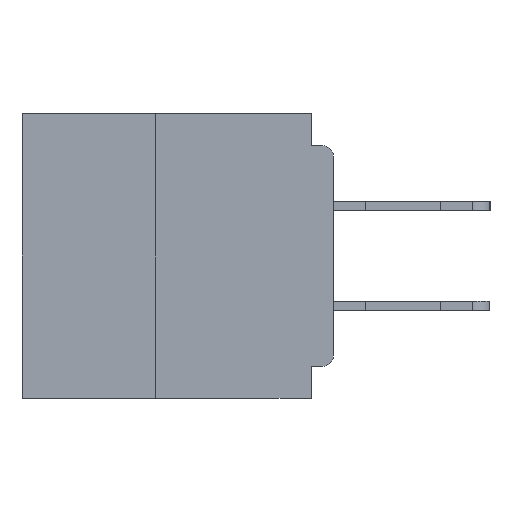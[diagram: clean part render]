
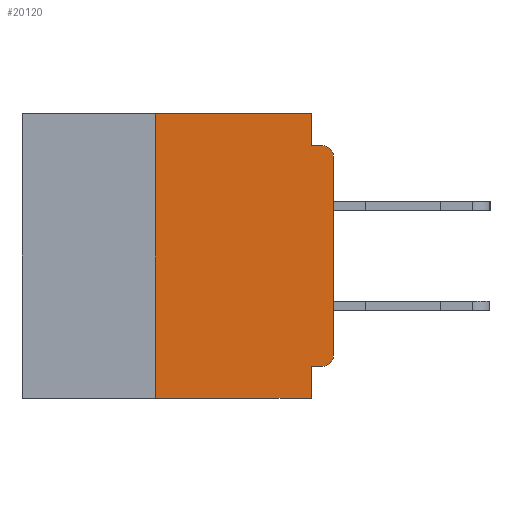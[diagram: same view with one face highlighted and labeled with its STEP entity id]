
A CAD part, left-side view. The second image highlights one B-rep face of the part: STEP entity #20120.
In plain terms, the highlighted planar face has unit normal (-1, 0, 0).
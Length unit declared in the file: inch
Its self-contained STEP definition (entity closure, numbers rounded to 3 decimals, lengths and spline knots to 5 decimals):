
#672 = CARTESIAN_POINT ( 'NONE',  ( 0., 0., -0.06 ) ) ;
#789 = CARTESIAN_POINT ( 'NONE',  ( 0., 0.031, -0.045 ) ) ;
#792 = EDGE_CURVE ( 'NONE', #22441, #14291, #31582, .T. ) ;
#2682 = EDGE_CURVE ( 'NONE', #5539, #14291, #34932, .T. ) ;
#2962 = DIRECTION ( 'NONE',  ( 0., 1., 0. ) ) ;
#2996 = LINE ( 'NONE', #38548, #36678 ) ;
#3114 = EDGE_LOOP ( 'NONE', ( #33244, #31197, #29555, #33017, #8066, #11037, #27765, #27818, #9573, #27859 ) ) ;
#3295 = CARTESIAN_POINT ( 'NONE',  ( 0., 0.437, 0. ) ) ;
#4267 = DIRECTION ( 'NONE',  ( 0., 0., -1. ) ) ;
#4683 = VERTEX_POINT ( 'NONE', #6016 ) ;
#4713 = AXIS2_PLACEMENT_3D ( 'NONE', #6894, #29725, #10182 ) ;
#5215 = VECTOR ( 'NONE', #4267, 39.37008 ) ;
#5427 = DIRECTION ( 'NONE',  ( 0., 0., -1. ) ) ;
#5489 = DIRECTION ( 'NONE',  ( -1., 0., 0. ) ) ;
#5539 = VERTEX_POINT ( 'NONE', #672 ) ;
#5543 = CARTESIAN_POINT ( 'NONE',  ( 0., 0.015, -0.06 ) ) ;
#5824 = CARTESIAN_POINT ( 'NONE',  ( 0., 0.25, -0.4 ) ) ;
#6016 = CARTESIAN_POINT ( 'NONE',  ( 0., 0.25, 0. ) ) ;
#6232 = VERTEX_POINT ( 'NONE', #18194 ) ;
#6638 = DIRECTION ( 'NONE',  ( 1., 0., 0. ) ) ;
#6881 = CARTESIAN_POINT ( 'NONE',  ( 0., 0., -0.045 ) ) ;
#6894 = CARTESIAN_POINT ( 'NONE',  ( 0., 0.015, -0.34 ) ) ;
#6960 = CARTESIAN_POINT ( 'NONE',  ( 0., 0.031, -0.4 ) ) ;
#8066 = ORIENTED_EDGE ( 'NONE', *, *, #27387, .F. ) ;
#9132 = VERTEX_POINT ( 'NONE', #11301 ) ;
#9573 = ORIENTED_EDGE ( 'NONE', *, *, #10696, .F. ) ;
#10182 = DIRECTION ( 'NONE',  ( 0., 0., -1. ) ) ;
#10696 = EDGE_CURVE ( 'NONE', #42075, #9132, #21358, .T. ) ;
#10853 = VECTOR ( 'NONE', #29791, 39.37008 ) ;
#11037 = ORIENTED_EDGE ( 'NONE', *, *, #32215, .F. ) ;
#11206 = VERTEX_POINT ( 'NONE', #5824 ) ;
#11301 = CARTESIAN_POINT ( 'NONE',  ( 0., 0.031, -0.355 ) ) ;
#11673 = AXIS2_PLACEMENT_3D ( 'NONE', #5543, #5489, #5427 ) ;
#11776 = DIRECTION ( 'NONE',  ( 0., -1., 0. ) ) ;
#12519 = CARTESIAN_POINT ( 'NONE',  ( 0., 0.015, -0.045 ) ) ;
#13280 = DIRECTION ( 'NONE',  ( 0., -1., 0. ) ) ;
#14195 = CARTESIAN_POINT ( 'NONE',  ( 0., 0.031, 0. ) ) ;
#14291 = VERTEX_POINT ( 'NONE', #12519 ) ;
#15713 = CARTESIAN_POINT ( 'NONE',  ( 0., 0.015, -0.355 ) ) ;
#17928 = LINE ( 'NONE', #30684, #34190 ) ;
#18194 = CARTESIAN_POINT ( 'NONE',  ( 0., 0.031, 0. ) ) ;
#18549 = LINE ( 'NONE', #6960, #10853 ) ;
#19301 = CARTESIAN_POINT ( 'NONE',  ( 0., 0., -0.355 ) ) ;
#20120 = ADVANCED_FACE ( 'NONE', ( #40018 ), #26079, .F. ) ;
#21358 = LINE ( 'NONE', #19301, #28982 ) ;
#21625 = LINE ( 'NONE', #14195, #5215 ) ;
#22441 = VERTEX_POINT ( 'NONE', #789 ) ;
#24100 = EDGE_CURVE ( 'NONE', #42075, #29612, #40668, .T. ) ;
#24923 = AXIS2_PLACEMENT_3D ( 'NONE', #3295, #6638, #29472 ) ;
#26079 = PLANE ( 'NONE',  #24923 ) ;
#26408 = CARTESIAN_POINT ( 'NONE',  ( 0., 0.437, 0. ) ) ;
#27348 = VECTOR ( 'NONE', #13280, 39.37008 ) ;
#27387 = EDGE_CURVE ( 'NONE', #4683, #6232, #37942, .T. ) ;
#27765 = ORIENTED_EDGE ( 'NONE', *, *, #38366, .T. ) ;
#27818 = ORIENTED_EDGE ( 'NONE', *, *, #37207, .F. ) ;
#27859 = ORIENTED_EDGE ( 'NONE', *, *, #24100, .T. ) ;
#28982 = VECTOR ( 'NONE', #2962, 39.37008 ) ;
#29472 = DIRECTION ( 'NONE',  ( 0., 0., -1. ) ) ;
#29555 = ORIENTED_EDGE ( 'NONE', *, *, #792, .F. ) ;
#29612 = VERTEX_POINT ( 'NONE', #42108 ) ;
#29725 = DIRECTION ( 'NONE',  ( -1., 0., 0. ) ) ;
#29791 = DIRECTION ( 'NONE',  ( 0., 0., -1. ) ) ;
#30131 = CARTESIAN_POINT ( 'NONE',  ( 0., 0.25, -0.4 ) ) ;
#30171 = EDGE_CURVE ( 'NONE', #29612, #5539, #2996, .T. ) ;
#30441 = VECTOR ( 'NONE', #36765, 39.37008 ) ;
#30684 = CARTESIAN_POINT ( 'NONE',  ( 0., 0.437, -0.4 ) ) ;
#31197 = ORIENTED_EDGE ( 'NONE', *, *, #2682, .T. ) ;
#31466 = LINE ( 'NONE', #30131, #30441 ) ;
#31582 = LINE ( 'NONE', #6881, #39118 ) ;
#32092 = VERTEX_POINT ( 'NONE', #32972 ) ;
#32215 = EDGE_CURVE ( 'NONE', #11206, #4683, #31466, .T. ) ;
#32972 = CARTESIAN_POINT ( 'NONE',  ( 0., 0.031, -0.4 ) ) ;
#33017 = ORIENTED_EDGE ( 'NONE', *, *, #41302, .F. ) ;
#33244 = ORIENTED_EDGE ( 'NONE', *, *, #30171, .T. ) ;
#33922 = DIRECTION ( 'NONE',  ( 0., -1., 0. ) ) ;
#34190 = VECTOR ( 'NONE', #33922, 39.37008 ) ;
#34932 = CIRCLE ( 'NONE', #11673, 0.015 ) ;
#35451 = DIRECTION ( 'NONE',  ( 0., 0., 1. ) ) ;
#36678 = VECTOR ( 'NONE', #35451, 39.37008 ) ;
#36765 = DIRECTION ( 'NONE',  ( 0., 0., 1. ) ) ;
#37207 = EDGE_CURVE ( 'NONE', #9132, #32092, #18549, .T. ) ;
#37942 = LINE ( 'NONE', #26408, #27348 ) ;
#38366 = EDGE_CURVE ( 'NONE', #11206, #32092, #17928, .T. ) ;
#38548 = CARTESIAN_POINT ( 'NONE',  ( 0., 0., 0. ) ) ;
#39118 = VECTOR ( 'NONE', #11776, 39.37008 ) ;
#40018 = FACE_OUTER_BOUND ( 'NONE', #3114, .T. ) ;
#40668 = CIRCLE ( 'NONE', #4713, 0.015 ) ;
#41302 = EDGE_CURVE ( 'NONE', #6232, #22441, #21625, .T. ) ;
#42075 = VERTEX_POINT ( 'NONE', #15713 ) ;
#42108 = CARTESIAN_POINT ( 'NONE',  ( 0., 0., -0.34 ) ) ;
